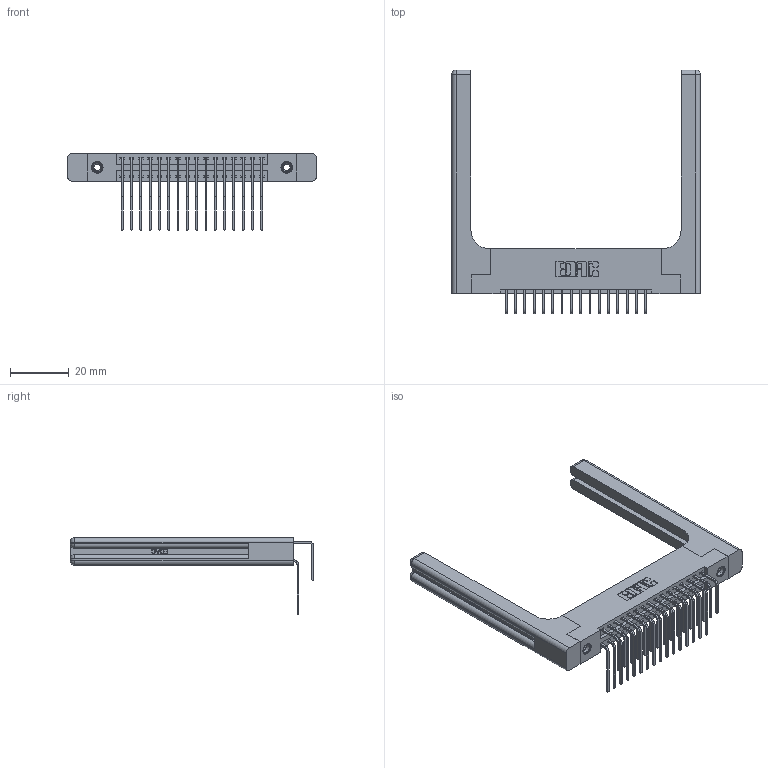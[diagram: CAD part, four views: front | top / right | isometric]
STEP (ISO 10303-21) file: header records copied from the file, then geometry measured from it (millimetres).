
FILE_DESCRIPTION (( 'STEP AP203' ), '1' );
FILE_NAME ('396-032-558-258.STEP', '2019-11-03T06:40:26', ( '' ), ( '' ), 'SwSTEP 2.0', 'SolidWorks 2016', '' );
FILE_SCHEMA (( 'CONFIG_CONTROL_DESIGN' ));
Length unit declared in the file: inch
Products named in the file (6): 346 Part_Flush Mounting Lugs - 0.156 Dia-TH; 396-032-558-258; 346-220-058_345-220-058; 345-292-001_558 559 Tail - 1; 345-250-001_345-250-001-102; 345-292-001_558 Tail - 2
Assembly tree (37 placements, depth 2):
  396-032-558-258
    346 Part_Flush Mounting Lugs - 0.156 Dia-TH
    345-292-001_558 559 Tail - 1  x16
    345-292-001_558 Tail - 2  x16
    345-250-001_345-250-001-102  x2
    346-220-058_345-220-058  x2
Bounding box: 84.86 x 83.12 x 26.16 mm (x, y, z)
Volume: 15751.9 mm3; surface area: 16800.5 mm2
Topology: 37 solids, 37 shells, 2106 faces, 6147 edges, 4034 vertices
Faces by surface type: plane 1408, cylinder 638, bspline 36, cone 12, sphere 8, torus 4
Entity records: 20908 total; most frequent: CARTESIAN_POINT 4540, ORIENTED_EDGE 3220, DIRECTION 2958, EDGE_CURVE 1610, LINE 1282, VECTOR 1282, VERTEX_POINT 1062, AXIS2_PLACEMENT_3D 838
